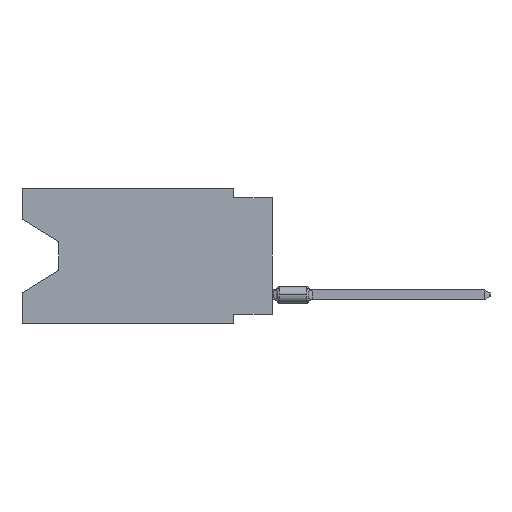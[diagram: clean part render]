
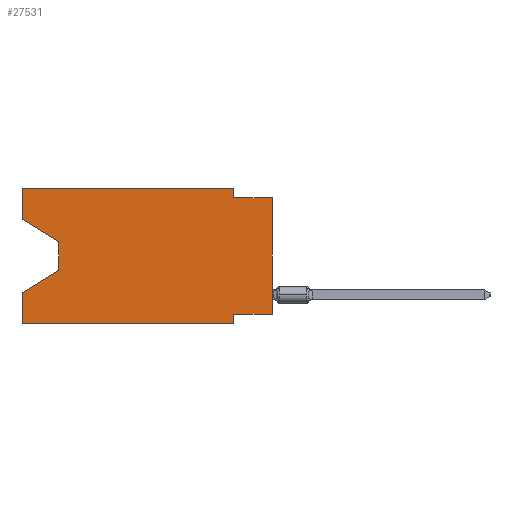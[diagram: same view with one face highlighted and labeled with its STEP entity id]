
A CAD part, left-side view. The second image highlights one B-rep face of the part: STEP entity #27531.
In plain terms, the highlighted planar face has unit normal (-1, 0, 0).
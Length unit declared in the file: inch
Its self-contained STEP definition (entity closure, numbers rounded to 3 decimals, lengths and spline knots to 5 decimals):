
#379 = ORIENTED_EDGE ( 'NONE', *, *, #17800, .F. ) ;
#760 = CARTESIAN_POINT ( 'NONE',  ( 0., 0.55, -0.138 ) ) ;
#1280 = EDGE_CURVE ( 'NONE', #22519, #44897, #25547, .T. ) ;
#1340 = DIRECTION ( 'NONE',  ( 0., 1., 0. ) ) ;
#3287 = ORIENTED_EDGE ( 'NONE', *, *, #51026, .T. ) ;
#3366 = DIRECTION ( 'NONE',  ( 0., 0., -1. ) ) ;
#3607 = VERTEX_POINT ( 'NONE', #31208 ) ;
#3693 = VECTOR ( 'NONE', #7520, 39.37008 ) ;
#4073 = VERTEX_POINT ( 'NONE', #40290 ) ;
#4561 = ORIENTED_EDGE ( 'NONE', *, *, #1280, .T. ) ;
#4700 = DIRECTION ( 'NONE',  ( 0., -0.855, -0.519 ) ) ;
#6576 = LINE ( 'NONE', #25828, #40182 ) ;
#7330 = CARTESIAN_POINT ( 'NONE',  ( 0., 0.1, 0. ) ) ;
#7520 = DIRECTION ( 'NONE',  ( 0., -1., 0. ) ) ;
#7621 = EDGE_CURVE ( 'NONE', #7625, #51690, #17499, .T. ) ;
#7625 = VERTEX_POINT ( 'NONE', #42828 ) ;
#7840 = DIRECTION ( 'NONE',  ( 0., -1., 0. ) ) ;
#8321 = CARTESIAN_POINT ( 'NONE',  ( 0., 0.645, 0. ) ) ;
#8533 = EDGE_CURVE ( 'NONE', #13869, #44698, #42955, .T. ) ;
#8656 = EDGE_CURVE ( 'NONE', #30772, #13869, #52147, .T. ) ;
#8670 = VECTOR ( 'NONE', #38341, 39.37008 ) ;
#9197 = LINE ( 'NONE', #44805, #33213 ) ;
#9335 = CARTESIAN_POINT ( 'NONE',  ( 0., 0., 0. ) ) ;
#9785 = CARTESIAN_POINT ( 'NONE',  ( 0., 0.1, 0. ) ) ;
#11501 = ORIENTED_EDGE ( 'NONE', *, *, #39537, .F. ) ;
#11833 = EDGE_CURVE ( 'NONE', #4073, #3607, #21894, .T. ) ;
#12032 = FACE_OUTER_BOUND ( 'NONE', #25822, .T. ) ;
#12347 = ORIENTED_EDGE ( 'NONE', *, *, #7621, .F. ) ;
#12416 = AXIS2_PLACEMENT_3D ( 'NONE', #8321, #16499, #24912 ) ;
#13005 = EDGE_CURVE ( 'NONE', #4073, #14242, #25669, .T. ) ;
#13869 = VERTEX_POINT ( 'NONE', #9785 ) ;
#14234 = EDGE_CURVE ( 'NONE', #44897, #51690, #9197, .T. ) ;
#14242 = VERTEX_POINT ( 'NONE', #44539 ) ;
#14667 = VECTOR ( 'NONE', #7840, 39.37008 ) ;
#15141 = CARTESIAN_POINT ( 'NONE',  ( 0., 0.1, -0.35 ) ) ;
#16499 = DIRECTION ( 'NONE',  ( 1., 0., 0. ) ) ;
#17499 = LINE ( 'NONE', #38595, #8670 ) ;
#17800 = EDGE_CURVE ( 'NONE', #20502, #30772, #24045, .T. ) ;
#18517 = ORIENTED_EDGE ( 'NONE', *, *, #14234, .T. ) ;
#19598 = DIRECTION ( 'NONE',  ( 0., 0., 1. ) ) ;
#19643 = VECTOR ( 'NONE', #49160, 39.37008 ) ;
#19947 = PLANE ( 'NONE',  #12416 ) ;
#20332 = CARTESIAN_POINT ( 'NONE',  ( 0., 0.1, -0.35 ) ) ;
#20502 = VERTEX_POINT ( 'NONE', #40295 ) ;
#21470 = ORIENTED_EDGE ( 'NONE', *, *, #11833, .F. ) ;
#21894 = LINE ( 'NONE', #37998, #34686 ) ;
#22519 = VERTEX_POINT ( 'NONE', #28360 ) ;
#23582 = CARTESIAN_POINT ( 'NONE',  ( 0., 0.55, -0.212 ) ) ;
#24045 = LINE ( 'NONE', #36197, #42070 ) ;
#24912 = DIRECTION ( 'NONE',  ( 0., 0., -1. ) ) ;
#24996 = DIRECTION ( 'NONE',  ( 0., 0.855, -0.519 ) ) ;
#25547 = LINE ( 'NONE', #760, #46484 ) ;
#25669 = LINE ( 'NONE', #9335, #19643 ) ;
#25822 = EDGE_LOOP ( 'NONE', ( #3287, #4561, #18517, #12347, #43245, #11501, #21470, #46429, #45513, #33920, #48917, #379 ) ) ;
#25828 = CARTESIAN_POINT ( 'NONE',  ( 0., 0.645, -0.35 ) ) ;
#26938 = EDGE_CURVE ( 'NONE', #7625, #32813, #6576, .T. ) ;
#27531 = ADVANCED_FACE ( 'NONE', ( #12032 ), #19947, .F. ) ;
#27647 = CARTESIAN_POINT ( 'NONE',  ( 0., 0.645, 0. ) ) ;
#28148 = CARTESIAN_POINT ( 'NONE',  ( 0., 0.645, 0. ) ) ;
#28339 = LINE ( 'NONE', #40467, #3693 ) ;
#28360 = CARTESIAN_POINT ( 'NONE',  ( 0., 0.55, -0.138 ) ) ;
#29266 = DIRECTION ( 'NONE',  ( 0., 0., -1. ) ) ;
#30772 = VERTEX_POINT ( 'NONE', #27647 ) ;
#31208 = CARTESIAN_POINT ( 'NONE',  ( 0., 0.1, -0.325 ) ) ;
#32672 = LINE ( 'NONE', #49004, #39126 ) ;
#32813 = VERTEX_POINT ( 'NONE', #15141 ) ;
#33213 = VECTOR ( 'NONE', #24996, 39.37008 ) ;
#33920 = ORIENTED_EDGE ( 'NONE', *, *, #8533, .F. ) ;
#34686 = VECTOR ( 'NONE', #1340, 39.37008 ) ;
#35472 = CARTESIAN_POINT ( 'NONE',  ( 0., 0.645, -0.26975 ) ) ;
#36197 = CARTESIAN_POINT ( 'NONE',  ( 0., 0.645, 0. ) ) ;
#37998 = CARTESIAN_POINT ( 'NONE',  ( 0., 0., -0.325 ) ) ;
#38341 = DIRECTION ( 'NONE',  ( 0., 0., 1. ) ) ;
#38595 = CARTESIAN_POINT ( 'NONE',  ( 0., 0.645, 0. ) ) ;
#39126 = VECTOR ( 'NONE', #4700, 39.37008 ) ;
#39537 = EDGE_CURVE ( 'NONE', #3607, #32813, #43831, .T. ) ;
#40182 = VECTOR ( 'NONE', #41941, 39.37008 ) ;
#40290 = CARTESIAN_POINT ( 'NONE',  ( 0., 0., -0.325 ) ) ;
#40295 = CARTESIAN_POINT ( 'NONE',  ( 0., 0.645, -0.08025 ) ) ;
#40467 = CARTESIAN_POINT ( 'NONE',  ( 0., 0., -0.025 ) ) ;
#40927 = DIRECTION ( 'NONE',  ( 0., 0., -1. ) ) ;
#41617 = VECTOR ( 'NONE', #3366, 39.37008 ) ;
#41856 = CARTESIAN_POINT ( 'NONE',  ( 0., 0.1, -0.025 ) ) ;
#41940 = EDGE_CURVE ( 'NONE', #44698, #14242, #28339, .T. ) ;
#41941 = DIRECTION ( 'NONE',  ( 0., -1., 0. ) ) ;
#42070 = VECTOR ( 'NONE', #19598, 39.37008 ) ;
#42265 = VECTOR ( 'NONE', #40927, 39.37008 ) ;
#42828 = CARTESIAN_POINT ( 'NONE',  ( 0., 0.645, -0.35 ) ) ;
#42955 = LINE ( 'NONE', #7330, #41617 ) ;
#43245 = ORIENTED_EDGE ( 'NONE', *, *, #26938, .T. ) ;
#43831 = LINE ( 'NONE', #20332, #42265 ) ;
#44539 = CARTESIAN_POINT ( 'NONE',  ( 0., 0., -0.025 ) ) ;
#44698 = VERTEX_POINT ( 'NONE', #41856 ) ;
#44805 = CARTESIAN_POINT ( 'NONE',  ( 0., 0.55, -0.212 ) ) ;
#44897 = VERTEX_POINT ( 'NONE', #23582 ) ;
#45513 = ORIENTED_EDGE ( 'NONE', *, *, #41940, .F. ) ;
#46429 = ORIENTED_EDGE ( 'NONE', *, *, #13005, .T. ) ;
#46484 = VECTOR ( 'NONE', #29266, 39.37008 ) ;
#48917 = ORIENTED_EDGE ( 'NONE', *, *, #8656, .F. ) ;
#49004 = CARTESIAN_POINT ( 'NONE',  ( 0., 0.645, -0.08025 ) ) ;
#49160 = DIRECTION ( 'NONE',  ( 0., 0., 1. ) ) ;
#51026 = EDGE_CURVE ( 'NONE', #20502, #22519, #32672, .T. ) ;
#51690 = VERTEX_POINT ( 'NONE', #35472 ) ;
#52147 = LINE ( 'NONE', #28148, #14667 ) ;
